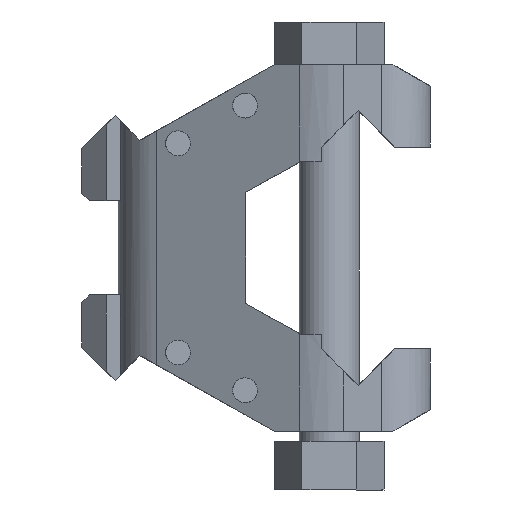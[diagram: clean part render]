
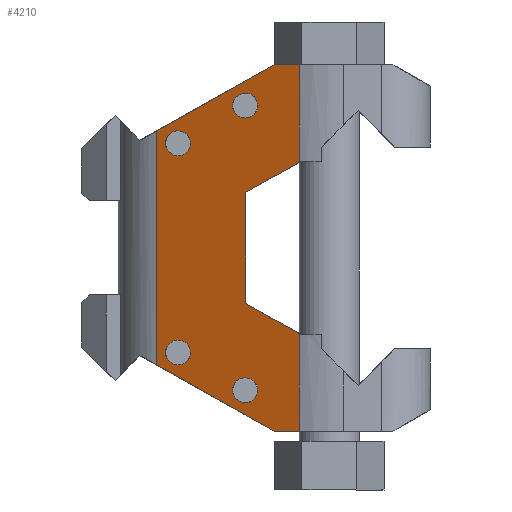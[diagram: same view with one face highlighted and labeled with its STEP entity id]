
A CAD part, left-side view. The second image highlights one B-rep face of the part: STEP entity #4210.
In plain terms, the highlighted planar face has unit normal (-0.904, 0.428, 0).
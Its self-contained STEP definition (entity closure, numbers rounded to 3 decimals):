
#57=FACE_BOUND('',#526,.T.);
#58=FACE_BOUND('',#527,.T.);
#59=FACE_BOUND('',#528,.T.);
#60=FACE_BOUND('',#529,.T.);
#104=PLANE('',#4488);
#294=FACE_OUTER_BOUND('',#525,.T.);
#525=EDGE_LOOP('',(#3103,#3104,#3105,#3106,#3107,#3108,#3109,#3110,#3111,
#3112));
#526=EDGE_LOOP('',(#3113));
#527=EDGE_LOOP('',(#3114));
#528=EDGE_LOOP('',(#3115));
#529=EDGE_LOOP('',(#3116));
#754=ELLIPSE('',#4489,1.134,1.025);
#755=ELLIPSE('',#4490,1.134,1.025);
#756=ELLIPSE('',#4491,1.134,1.025);
#757=ELLIPSE('',#4492,1.134,1.025);
#800=LINE('',#5974,#1296);
#819=LINE('',#6037,#1315);
#882=LINE('',#6189,#1378);
#913=LINE('',#6255,#1409);
#919=LINE('',#6360,#1415);
#920=LINE('',#6362,#1416);
#921=LINE('',#6364,#1417);
#922=LINE('',#6366,#1418);
#923=LINE('',#6368,#1419);
#924=LINE('',#6369,#1420);
#1296=VECTOR('',#4792,10.);
#1315=VECTOR('',#4847,10.);
#1378=VECTOR('',#4972,10.);
#1409=VECTOR('',#5013,10.);
#1415=VECTOR('',#5023,10.);
#1416=VECTOR('',#5024,10.);
#1417=VECTOR('',#5025,10.);
#1418=VECTOR('',#5026,10.);
#1419=VECTOR('',#5027,10.);
#1420=VECTOR('',#5028,10.);
#1859=VERTEX_POINT('',#5971);
#1860=VERTEX_POINT('',#5973);
#1885=VERTEX_POINT('',#6034);
#1886=VERTEX_POINT('',#6036);
#1943=VERTEX_POINT('',#6186);
#1944=VERTEX_POINT('',#6188);
#1984=VERTEX_POINT('',#6361);
#1985=VERTEX_POINT('',#6363);
#1986=VERTEX_POINT('',#6365);
#1987=VERTEX_POINT('',#6367);
#1988=VERTEX_POINT('',#6370);
#1989=VERTEX_POINT('',#6372);
#1990=VERTEX_POINT('',#6374);
#1991=VERTEX_POINT('',#6376);
#2280=EDGE_CURVE('',#1859,#1860,#800,.T.);
#2311=EDGE_CURVE('',#1885,#1886,#819,.T.);
#2385=EDGE_CURVE('',#1943,#1944,#882,.T.);
#2419=EDGE_CURVE('',#1944,#1885,#913,.T.);
#2430=EDGE_CURVE('',#1860,#1943,#919,.T.);
#2431=EDGE_CURVE('',#1984,#1859,#920,.T.);
#2432=EDGE_CURVE('',#1985,#1984,#921,.T.);
#2433=EDGE_CURVE('',#1986,#1985,#922,.T.);
#2434=EDGE_CURVE('',#1987,#1986,#923,.T.);
#2435=EDGE_CURVE('',#1886,#1987,#924,.T.);
#2436=EDGE_CURVE('',#1988,#1988,#754,.T.);
#2437=EDGE_CURVE('',#1989,#1989,#755,.T.);
#2438=EDGE_CURVE('',#1990,#1990,#756,.T.);
#2439=EDGE_CURVE('',#1991,#1991,#757,.T.);
#3103=ORIENTED_EDGE('',*,*,#2385,.F.);
#3104=ORIENTED_EDGE('',*,*,#2430,.F.);
#3105=ORIENTED_EDGE('',*,*,#2280,.F.);
#3106=ORIENTED_EDGE('',*,*,#2431,.F.);
#3107=ORIENTED_EDGE('',*,*,#2432,.F.);
#3108=ORIENTED_EDGE('',*,*,#2433,.F.);
#3109=ORIENTED_EDGE('',*,*,#2434,.F.);
#3110=ORIENTED_EDGE('',*,*,#2435,.F.);
#3111=ORIENTED_EDGE('',*,*,#2311,.F.);
#3112=ORIENTED_EDGE('',*,*,#2419,.F.);
#3113=ORIENTED_EDGE('',*,*,#2436,.F.);
#3114=ORIENTED_EDGE('',*,*,#2437,.F.);
#3115=ORIENTED_EDGE('',*,*,#2438,.F.);
#3116=ORIENTED_EDGE('',*,*,#2439,.F.);
#4210=ADVANCED_FACE('',(#294,#57,#58,#59,#60),#104,.F.);
#4488=AXIS2_PLACEMENT_3D('',#6359,#5021,#5022);
#4489=AXIS2_PLACEMENT_3D('',#6371,#5029,#5030);
#4490=AXIS2_PLACEMENT_3D('',#6373,#5031,#5032);
#4491=AXIS2_PLACEMENT_3D('',#6375,#5033,#5034);
#4492=AXIS2_PLACEMENT_3D('',#6377,#5035,#5036);
#4792=DIRECTION('',(0.428,0.904,0.));
#4847=DIRECTION('',(-0.428,-0.904,0.));
#4972=DIRECTION('',(0.,0.,1.));
#5013=DIRECTION('',(-0.381,-0.806,0.453));
#5021=DIRECTION('center_axis',(0.904,-0.428,0.));
#5022=DIRECTION('ref_axis',(0.428,0.904,0.));
#5023=DIRECTION('',(0.381,0.806,0.453));
#5024=DIRECTION('',(0.,0.,-1.));
#5025=DIRECTION('',(-0.381,-0.806,-0.453));
#5026=DIRECTION('',(0.,0.,-1.));
#5027=DIRECTION('',(0.381,0.806,-0.453));
#5028=DIRECTION('',(0.,0.,-1.));
#5029=DIRECTION('center_axis',(-0.904,0.428,0.));
#5030=DIRECTION('ref_axis',(0.428,0.904,0.));
#5031=DIRECTION('center_axis',(-0.904,0.428,0.));
#5032=DIRECTION('ref_axis',(0.428,0.904,0.));
#5033=DIRECTION('center_axis',(-0.904,0.428,0.));
#5034=DIRECTION('ref_axis',(0.428,0.904,0.));
#5035=DIRECTION('center_axis',(-0.904,0.428,0.));
#5036=DIRECTION('ref_axis',(0.428,0.904,0.));
#5971=CARTESIAN_POINT('',(14.005,189.815,149.934));
#5973=CARTESIAN_POINT('',(14.965,191.844,149.934));
#5974=CARTESIAN_POINT('',(16.126,194.299,149.934));
#6034=CARTESIAN_POINT('',(14.965,191.844,180.107));
#6036=CARTESIAN_POINT('',(14.005,189.815,180.107));
#6037=CARTESIAN_POINT('',(18.006,198.273,180.107));
#6186=CARTESIAN_POINT('',(19.567,201.573,155.409));
#6188=CARTESIAN_POINT('',(19.567,201.573,174.632));
#6189=CARTESIAN_POINT('',(19.567,201.573,155.546));
#6255=CARTESIAN_POINT('',(22.534,207.844,171.103));
#6359=CARTESIAN_POINT('Origin',(13.189,188.09,149.934));
#6360=CARTESIAN_POINT('',(17.381,196.951,152.808));
#6361=CARTESIAN_POINT('',(14.005,189.815,157.972));
#6362=CARTESIAN_POINT('',(14.005,189.815,152.029));
#6363=CARTESIAN_POINT('',(16.096,194.235,160.46));
#6364=CARTESIAN_POINT('',(17.516,197.237,162.149));
#6365=CARTESIAN_POINT('',(16.096,194.235,169.582));
#6366=CARTESIAN_POINT('',(16.096,194.235,161.477));
#6367=CARTESIAN_POINT('',(14.005,189.815,172.069));
#6368=CARTESIAN_POINT('',(18.771,199.89,166.399));
#6369=CARTESIAN_POINT('',(14.005,189.815,152.029));
#6370=CARTESIAN_POINT('',(18.24,198.768,156.416));
#6371=CARTESIAN_POINT('Origin',(18.725,199.793,156.416));
#6372=CARTESIAN_POINT('',(15.63,193.25,176.731));
#6373=CARTESIAN_POINT('Origin',(16.115,194.275,176.731));
#6374=CARTESIAN_POINT('',(15.63,193.25,153.31));
#6375=CARTESIAN_POINT('Origin',(16.115,194.275,153.31));
#6376=CARTESIAN_POINT('',(18.24,198.768,173.625));
#6377=CARTESIAN_POINT('Origin',(18.725,199.793,173.625));
